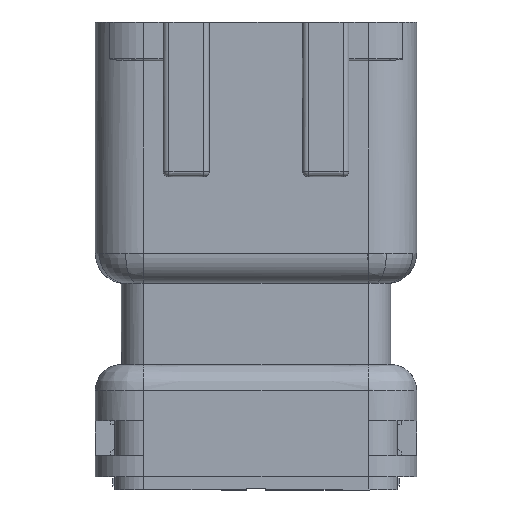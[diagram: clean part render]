
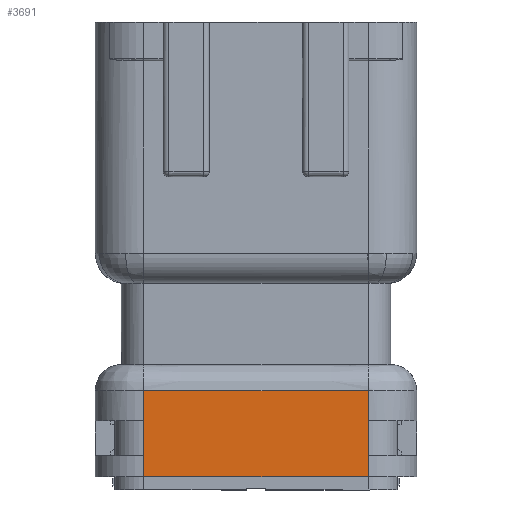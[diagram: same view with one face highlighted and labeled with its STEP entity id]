
A CAD part, front view. The second image highlights one B-rep face of the part: STEP entity #3691.
In plain terms, the highlighted planar face has unit normal (0, -1, 0).
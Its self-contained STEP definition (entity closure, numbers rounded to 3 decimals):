
#88 = DIRECTION ( 'NONE',  ( 0., 0., 1. ) ) ;
#523 = LINE ( 'NONE', #16092, #14559 ) ;
#775 = LINE ( 'NONE', #5750, #12121 ) ;
#1039 = VECTOR ( 'NONE', #20625, 1000. ) ;
#1777 = B_SPLINE_CURVE_WITH_KNOTS ( 'NONE', 3,
 ( #15905, #7222, #14088, #12726 ),
 .UNSPECIFIED., .F., .F.,
 ( 4, 4 ),
 ( 0., 1. ),
 .UNSPECIFIED. ) ;
#2372 = CARTESIAN_POINT ( 'NONE',  ( -5.8, -4., -10. ) ) ;
#2562 = CARTESIAN_POINT ( 'NONE',  ( -5.8, -4., -5.55 ) ) ;
#3179 = VERTEX_POINT ( 'NONE', #5470 ) ;
#3691 = ADVANCED_FACE ( 'NONE', ( #18286 ), #10947, .F. ) ;
#3713 = VECTOR ( 'NONE', #4836, 1000. ) ;
#4269 = LINE ( 'NONE', #14332, #5170 ) ;
#4836 = DIRECTION ( 'NONE',  ( -1., 0., 0. ) ) ;
#5170 = VECTOR ( 'NONE', #19535, 1000. ) ;
#5270 = EDGE_CURVE ( 'NONE', #18018, #11743, #19430, .T. ) ;
#5470 = CARTESIAN_POINT ( 'NONE',  ( -5.8, -4., -8.9 ) ) ;
#5664 = EDGE_CURVE ( 'NONE', #10348, #8530, #775, .T. ) ;
#5750 = CARTESIAN_POINT ( 'NONE',  ( -5.8, -4., -10. ) ) ;
#5970 = DIRECTION ( 'NONE',  ( 0., 0., 1. ) ) ;
#6273 = CARTESIAN_POINT ( 'NONE',  ( 5.8, -4., -5.55 ) ) ;
#6449 = EDGE_LOOP ( 'NONE', ( #8080, #14915, #11330, #11374, #13191, #18039, #15506, #15064 ) ) ;
#6863 = LINE ( 'NONE', #13726, #1039 ) ;
#7003 = CARTESIAN_POINT ( 'NONE',  ( -5.8, -4., -10. ) ) ;
#7081 = CARTESIAN_POINT ( 'NONE',  ( 5.8, -4., -7.1 ) ) ;
#7222 = CARTESIAN_POINT ( 'NONE',  ( 1.933, -4., -5.55 ) ) ;
#7509 = CARTESIAN_POINT ( 'NONE',  ( -5.8, -4., -7.1 ) ) ;
#8080 = ORIENTED_EDGE ( 'NONE', *, *, #13188, .T. ) ;
#8326 = VERTEX_POINT ( 'NONE', #7003 ) ;
#8342 = DIRECTION ( 'NONE',  ( 0., 0., 1. ) ) ;
#8439 = EDGE_CURVE ( 'NONE', #19852, #8530, #1777, .T. ) ;
#8530 = VERTEX_POINT ( 'NONE', #2562 ) ;
#9570 = AXIS2_PLACEMENT_3D ( 'NONE', #2372, #16143, #8342 ) ;
#9914 = EDGE_CURVE ( 'NONE', #18018, #8326, #15201, .T. ) ;
#10348 = VERTEX_POINT ( 'NONE', #7509 ) ;
#10683 = CARTESIAN_POINT ( 'NONE',  ( 5.8, -4., -10. ) ) ;
#10936 = CARTESIAN_POINT ( 'NONE',  ( 5.8, -4., -10. ) ) ;
#10947 = PLANE ( 'NONE',  #9570 ) ;
#11126 = CARTESIAN_POINT ( 'NONE',  ( 5.8, -4., -8.9 ) ) ;
#11330 = ORIENTED_EDGE ( 'NONE', *, *, #5664, .F. ) ;
#11374 = ORIENTED_EDGE ( 'NONE', *, *, #12111, .T. ) ;
#11716 = VECTOR ( 'NONE', #14227, 1000. ) ;
#11743 = VERTEX_POINT ( 'NONE', #11126 ) ;
#11945 = VERTEX_POINT ( 'NONE', #7081 ) ;
#12111 = EDGE_CURVE ( 'NONE', #10348, #3179, #523, .T. ) ;
#12121 = VECTOR ( 'NONE', #5970, 1000. ) ;
#12726 = CARTESIAN_POINT ( 'NONE',  ( -5.8, -4., -5.55 ) ) ;
#12800 = DIRECTION ( 'NONE',  ( 0., 0., -1. ) ) ;
#13188 = EDGE_CURVE ( 'NONE', #11945, #19852, #17334, .T. ) ;
#13191 = ORIENTED_EDGE ( 'NONE', *, *, #15708, .F. ) ;
#13726 = CARTESIAN_POINT ( 'NONE',  ( -5.8, -4., -10. ) ) ;
#14088 = CARTESIAN_POINT ( 'NONE',  ( -1.933, -4., -5.55 ) ) ;
#14227 = DIRECTION ( 'NONE',  ( 0., 0., 1. ) ) ;
#14332 = CARTESIAN_POINT ( 'NONE',  ( 5.8, -4., -7.1 ) ) ;
#14559 = VECTOR ( 'NONE', #12800, 1000. ) ;
#14915 = ORIENTED_EDGE ( 'NONE', *, *, #8439, .T. ) ;
#15064 = ORIENTED_EDGE ( 'NONE', *, *, #20450, .F. ) ;
#15201 = LINE ( 'NONE', #22223, #3713 ) ;
#15506 = ORIENTED_EDGE ( 'NONE', *, *, #5270, .T. ) ;
#15708 = EDGE_CURVE ( 'NONE', #8326, #3179, #6863, .T. ) ;
#15905 = CARTESIAN_POINT ( 'NONE',  ( 5.8, -4., -5.55 ) ) ;
#16092 = CARTESIAN_POINT ( 'NONE',  ( -5.8, -4., -7.1 ) ) ;
#16143 = DIRECTION ( 'NONE',  ( 0., 1., 0. ) ) ;
#17334 = LINE ( 'NONE', #10683, #21589 ) ;
#18018 = VERTEX_POINT ( 'NONE', #10936 ) ;
#18039 = ORIENTED_EDGE ( 'NONE', *, *, #9914, .F. ) ;
#18286 = FACE_OUTER_BOUND ( 'NONE', #6449, .T. ) ;
#19430 = LINE ( 'NONE', #19650, #11716 ) ;
#19535 = DIRECTION ( 'NONE',  ( 0., 0., -1. ) ) ;
#19650 = CARTESIAN_POINT ( 'NONE',  ( 5.8, -4., -10. ) ) ;
#19852 = VERTEX_POINT ( 'NONE', #6273 ) ;
#20450 = EDGE_CURVE ( 'NONE', #11945, #11743, #4269, .T. ) ;
#20625 = DIRECTION ( 'NONE',  ( 0., 0., 1. ) ) ;
#21589 = VECTOR ( 'NONE', #88, 1000. ) ;
#22223 = CARTESIAN_POINT ( 'NONE',  ( -5.8, -4., -10. ) ) ;
